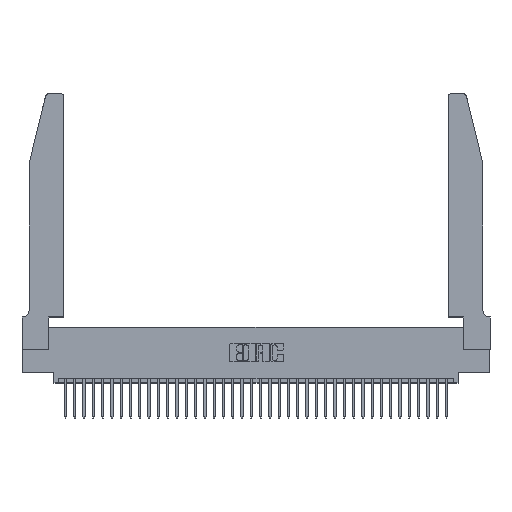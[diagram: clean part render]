
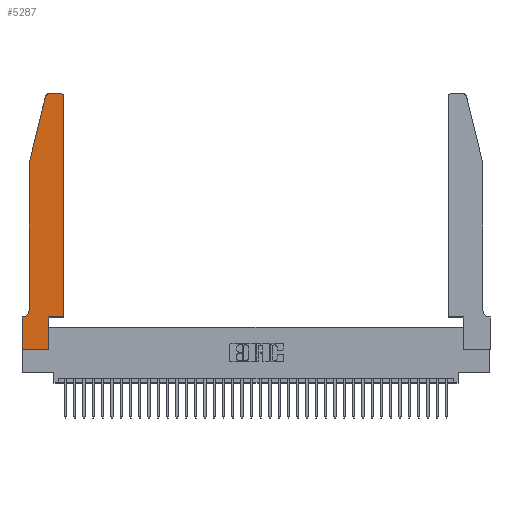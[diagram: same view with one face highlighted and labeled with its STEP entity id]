
A CAD part, top view. The second image highlights one B-rep face of the part: STEP entity #5287.
In plain terms, the highlighted planar face has unit normal (0, 0, 1).
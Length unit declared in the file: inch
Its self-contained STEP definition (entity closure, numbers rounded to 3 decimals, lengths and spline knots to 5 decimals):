
#428 = EDGE_CURVE ( 'NONE', #11698, #18694, #28827, .T. ) ;
#605 = VECTOR ( 'NONE', #17068, 39.37008 ) ;
#729 = ORIENTED_EDGE ( 'NONE', *, *, #34182, .T. ) ;
#2376 = ORIENTED_EDGE ( 'NONE', *, *, #428, .T. ) ;
#2684 = AXIS2_PLACEMENT_3D ( 'NONE', #26380, #17201, #17716 ) ;
#2730 = DIRECTION ( 'NONE',  ( 1., 0., 0. ) ) ;
#2906 = EDGE_CURVE ( 'NONE', #4437, #30786, #36664, .T. ) ;
#4437 = VERTEX_POINT ( 'NONE', #5000 ) ;
#4463 = ORIENTED_EDGE ( 'NONE', *, *, #24954, .T. ) ;
#4868 = CARTESIAN_POINT ( 'NONE',  ( 0.0755, 2., 0.37 ) ) ;
#4972 = VECTOR ( 'NONE', #2730, 39.37008 ) ;
#4989 = ORIENTED_EDGE ( 'NONE', *, *, #29306, .T. ) ;
#5000 = CARTESIAN_POINT ( 'NONE',  ( 0., 0.35, 0.37 ) ) ;
#5028 = EDGE_CURVE ( 'NONE', #36058, #18082, #32142, .T. ) ;
#5188 = VERTEX_POINT ( 'NONE', #11988 ) ;
#5194 = CARTESIAN_POINT ( 'NONE',  ( 0., 0., 0.37 ) ) ;
#5203 = VECTOR ( 'NONE', #7489, 39.37008 ) ;
#5287 = ADVANCED_FACE ( 'NONE', ( #30776 ), #12371, .T. ) ;
#5501 = LINE ( 'NONE', #4868, #16234 ) ;
#5601 = CARTESIAN_POINT ( 'NONE',  ( 0.0755, 0.42, 0.37 ) ) ;
#6797 = CARTESIAN_POINT ( 'NONE',  ( 0.2865, 0., 0.37 ) ) ;
#7489 = DIRECTION ( 'NONE',  ( 0., -1., 0. ) ) ;
#7634 = CARTESIAN_POINT ( 'NONE',  ( 0.4505, 0.35, 0.37 ) ) ;
#7647 = VECTOR ( 'NONE', #34175, 39.37008 ) ;
#7704 = ORIENTED_EDGE ( 'NONE', *, *, #9458, .T. ) ;
#7850 = ORIENTED_EDGE ( 'NONE', *, *, #18552, .T. ) ;
#8259 = EDGE_CURVE ( 'NONE', #30786, #23493, #23333, .T. ) ;
#8543 = LINE ( 'NONE', #14122, #605 ) ;
#8972 = ORIENTED_EDGE ( 'NONE', *, *, #26950, .T. ) ;
#9205 = CARTESIAN_POINT ( 'NONE',  ( 0., 0., 0.37 ) ) ;
#9458 = EDGE_CURVE ( 'NONE', #23493, #12723, #8543, .T. ) ;
#10014 = EDGE_LOOP ( 'NONE', ( #7850, #2376, #8972, #4463, #33814, #20319, #12610, #22992, #7704, #729, #4989, #27310 ) ) ;
#10195 = CARTESIAN_POINT ( 'NONE',  ( 0., 0., 0.37 ) ) ;
#10747 = CARTESIAN_POINT ( 'NONE',  ( 0.284, 2.75, 0.37 ) ) ;
#10907 = CARTESIAN_POINT ( 'NONE',  ( 0.4505, 2.72, 0.37 ) ) ;
#10972 = VERTEX_POINT ( 'NONE', #10907 ) ;
#11698 = VERTEX_POINT ( 'NONE', #10747 ) ;
#11904 = LINE ( 'NONE', #21463, #26542 ) ;
#11988 = CARTESIAN_POINT ( 'NONE',  ( 0.4505, 0.35, 0.37 ) ) ;
#12370 = CARTESIAN_POINT ( 'NONE',  ( 0.2865, 0.35, 0.37 ) ) ;
#12371 = PLANE ( 'NONE',  #26728 ) ;
#12610 = ORIENTED_EDGE ( 'NONE', *, *, #2906, .T. ) ;
#12723 = VERTEX_POINT ( 'NONE', #12370 ) ;
#13220 = DIRECTION ( 'NONE',  ( 0., -1., 0. ) ) ;
#13596 = CARTESIAN_POINT ( 'NONE',  ( 0.0055, 0.35, 0.37 ) ) ;
#14122 = CARTESIAN_POINT ( 'NONE',  ( 0.2865, 0.35, 0.37 ) ) ;
#16234 = VECTOR ( 'NONE', #16836, 39.37008 ) ;
#16328 = EDGE_CURVE ( 'NONE', #10972, #27479, #24462, .T. ) ;
#16685 = CARTESIAN_POINT ( 'NONE',  ( 0.4205, 2.75, 0.37 ) ) ;
#16836 = DIRECTION ( 'NONE',  ( -0.239, -0.971, 0. ) ) ;
#16838 = DIRECTION ( 'NONE',  ( 0., 0., 1. ) ) ;
#16999 = VERTEX_POINT ( 'NONE', #20071 ) ;
#17068 = DIRECTION ( 'NONE',  ( 0., 1., 0. ) ) ;
#17165 = CARTESIAN_POINT ( 'NONE',  ( 0.0055, 0.42, 0.37 ) ) ;
#17201 = DIRECTION ( 'NONE',  ( 0., 0., 1. ) ) ;
#17399 = LINE ( 'NONE', #7634, #25138 ) ;
#17716 = DIRECTION ( 'NONE',  ( 1., 0., 0. ) ) ;
#18082 = VERTEX_POINT ( 'NONE', #13596 ) ;
#18284 = DIRECTION ( 'NONE',  ( 1., 0., 0. ) ) ;
#18552 = EDGE_CURVE ( 'NONE', #27479, #11698, #11904, .T. ) ;
#18560 = DIRECTION ( 'NONE',  ( -1., 0., 0. ) ) ;
#18654 = VECTOR ( 'NONE', #13220, 39.37008 ) ;
#18694 = VERTEX_POINT ( 'NONE', #21976 ) ;
#20071 = CARTESIAN_POINT ( 'NONE',  ( 0.0755, 2., 0.37 ) ) ;
#20084 = DIRECTION ( 'NONE',  ( -1., 0., 0. ) ) ;
#20319 = ORIENTED_EDGE ( 'NONE', *, *, #36401, .T. ) ;
#20523 = VECTOR ( 'NONE', #30443, 39.37008 ) ;
#20918 = LINE ( 'NONE', #22198, #5203 ) ;
#21424 = LINE ( 'NONE', #27557, #20523 ) ;
#21463 = CARTESIAN_POINT ( 'NONE',  ( 0.2605, 2.75, 0.37 ) ) ;
#21613 = LINE ( 'NONE', #31949, #4972 ) ;
#21976 = CARTESIAN_POINT ( 'NONE',  ( 0.25487, 2.72718, 0.37 ) ) ;
#22198 = CARTESIAN_POINT ( 'NONE',  ( 0.0755, 2., 0.37 ) ) ;
#22992 = ORIENTED_EDGE ( 'NONE', *, *, #8259, .T. ) ;
#23333 = LINE ( 'NONE', #5194, #7647 ) ;
#23493 = VERTEX_POINT ( 'NONE', #6797 ) ;
#24462 = CIRCLE ( 'NONE', #35799, 0.03 ) ;
#24954 = EDGE_CURVE ( 'NONE', #16999, #36058, #20918, .T. ) ;
#25138 = VECTOR ( 'NONE', #25287, 39.37008 ) ;
#25287 = DIRECTION ( 'NONE',  ( 0., 1., 0. ) ) ;
#26380 = CARTESIAN_POINT ( 'NONE',  ( 0.284, 2.72, 0.37 ) ) ;
#26542 = VECTOR ( 'NONE', #18560, 39.37008 ) ;
#26728 = AXIS2_PLACEMENT_3D ( 'NONE', #32665, #35527, #18284 ) ;
#26950 = EDGE_CURVE ( 'NONE', #18694, #16999, #5501, .T. ) ;
#27310 = ORIENTED_EDGE ( 'NONE', *, *, #16328, .T. ) ;
#27479 = VERTEX_POINT ( 'NONE', #16685 ) ;
#27557 = CARTESIAN_POINT ( 'NONE',  ( 0.0755, 0.35, 0.37 ) ) ;
#28827 = CIRCLE ( 'NONE', #2684, 0.03 ) ;
#29306 = EDGE_CURVE ( 'NONE', #5188, #10972, #17399, .T. ) ;
#30443 = DIRECTION ( 'NONE',  ( -1., 0., 0. ) ) ;
#30776 = FACE_OUTER_BOUND ( 'NONE', #10014, .T. ) ;
#30786 = VERTEX_POINT ( 'NONE', #9205 ) ;
#31268 = AXIS2_PLACEMENT_3D ( 'NONE', #17165, #37299, #20084 ) ;
#31949 = CARTESIAN_POINT ( 'NONE',  ( 0.4505, 0.35, 0.37 ) ) ;
#32142 = CIRCLE ( 'NONE', #31268, 0.07 ) ;
#32665 = CARTESIAN_POINT ( 'NONE',  ( 0., 0.35, 0.37 ) ) ;
#33814 = ORIENTED_EDGE ( 'NONE', *, *, #5028, .T. ) ;
#34116 = CARTESIAN_POINT ( 'NONE',  ( 0.4205, 2.72, 0.37 ) ) ;
#34175 = DIRECTION ( 'NONE',  ( 1., 0., 0. ) ) ;
#34182 = EDGE_CURVE ( 'NONE', #12723, #5188, #21613, .T. ) ;
#35527 = DIRECTION ( 'NONE',  ( 0., 0., 1. ) ) ;
#35799 = AXIS2_PLACEMENT_3D ( 'NONE', #34116, #16838, #36979 ) ;
#36058 = VERTEX_POINT ( 'NONE', #5601 ) ;
#36401 = EDGE_CURVE ( 'NONE', #18082, #4437, #21424, .T. ) ;
#36664 = LINE ( 'NONE', #10195, #18654 ) ;
#36979 = DIRECTION ( 'NONE',  ( 1., 0., 0. ) ) ;
#37299 = DIRECTION ( 'NONE',  ( 0., 0., -1. ) ) ;
